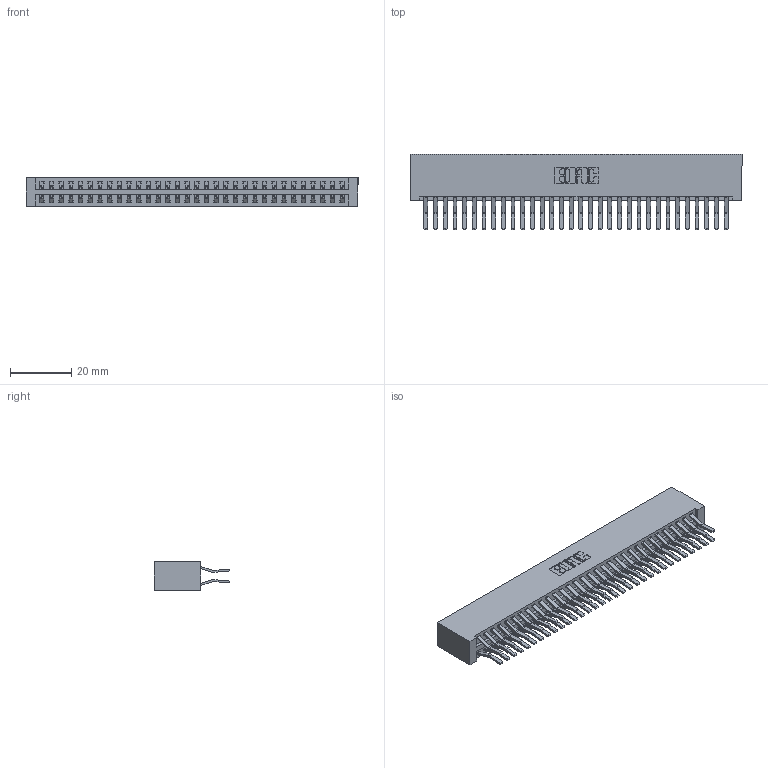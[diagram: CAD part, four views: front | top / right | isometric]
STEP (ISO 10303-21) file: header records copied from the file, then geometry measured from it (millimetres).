
FILE_DESCRIPTION (( 'STEP AP203' ), '1' );
FILE_NAME ('396-064-560-201.STEP', '2018-09-08T18:12:39', ( '' ), ( '' ), 'SwSTEP 2.0', 'SolidWorks 2016', '' );
FILE_SCHEMA (( 'CONFIG_CONTROL_DESIGN' ));
Length unit declared in the file: inch
Products named in the file (3): 346 Part_No Mounting Lugs; 345-292-001_560 Tail; 396-064-560-201
Assembly tree (65 placements, depth 2):
  396-064-560-201
    346 Part_No Mounting Lugs
    345-292-001_560 Tail  x64
Bounding box: 108.84 x 24.78 x 9.4 mm (x, y, z)
Volume: 11528.3 mm3; surface area: 16971.6 mm2
Topology: 65 solids, 65 shells, 3570 faces, 10609 edges, 6986 vertices
Faces by surface type: plane 2312, cylinder 1258
Entity records: 22041 total; most frequent: CARTESIAN_POINT 3644, ORIENTED_EDGE 3578, DIRECTION 3261, EDGE_CURVE 1789, LINE 1533, VECTOR 1533, VERTEX_POINT 1190, AXIS2_PLACEMENT_3D 864
